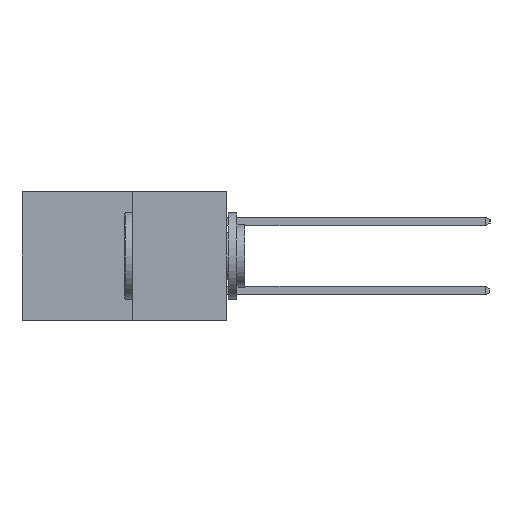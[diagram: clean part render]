
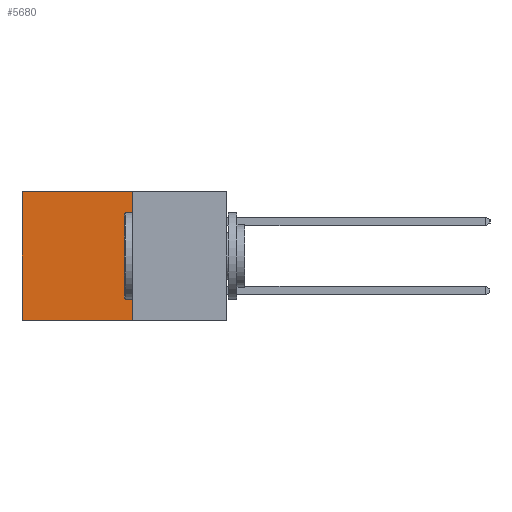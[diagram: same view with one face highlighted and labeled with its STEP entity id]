
A CAD part, left-side view. The second image highlights one B-rep face of the part: STEP entity #5680.
In plain terms, the highlighted planar face has unit normal (-1, 0, 0).
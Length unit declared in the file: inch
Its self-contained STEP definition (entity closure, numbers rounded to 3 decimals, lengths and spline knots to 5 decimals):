
#128 = DIRECTION ( 'NONE',  ( 0., 0., -1. ) ) ;
#725 = EDGE_LOOP ( 'NONE', ( #756, #8304, #2112, #6330 ) ) ;
#756 = ORIENTED_EDGE ( 'NONE', *, *, #2723, .T. ) ;
#822 = CARTESIAN_POINT ( 'NONE',  ( 0.277, 0.27, 0. ) ) ;
#1038 = FACE_OUTER_BOUND ( 'NONE', #725, .T. ) ;
#1588 = PLANE ( 'NONE',  #3209 ) ;
#1801 = VERTEX_POINT ( 'NONE', #3300 ) ;
#1844 = LINE ( 'NONE', #6355, #12254 ) ;
#2112 = ORIENTED_EDGE ( 'NONE', *, *, #11086, .F. ) ;
#2601 = DIRECTION ( 'NONE',  ( 0., 0., -1. ) ) ;
#2723 = EDGE_CURVE ( 'NONE', #10650, #10129, #11982, .T. ) ;
#3209 = AXIS2_PLACEMENT_3D ( 'NONE', #4567, #8621, #2601 ) ;
#3300 = CARTESIAN_POINT ( 'NONE',  ( 0.277, 0.27, 0. ) ) ;
#3557 = CARTESIAN_POINT ( 'NONE',  ( 0.277, 0.59, 0. ) ) ;
#4363 = VECTOR ( 'NONE', #128, 39.37008 ) ;
#4567 = CARTESIAN_POINT ( 'NONE',  ( 0.277, 0.27, -0.37 ) ) ;
#4668 = LINE ( 'NONE', #12145, #4363 ) ;
#5408 = LINE ( 'NONE', #822, #11142 ) ;
#5680 = ADVANCED_FACE ( 'NONE', ( #1038 ), #1588, .F. ) ;
#6177 = EDGE_CURVE ( 'NONE', #12588, #10129, #1844, .T. ) ;
#6278 = DIRECTION ( 'NONE',  ( 0., 0., -1. ) ) ;
#6330 = ORIENTED_EDGE ( 'NONE', *, *, #7717, .T. ) ;
#6355 = CARTESIAN_POINT ( 'NONE',  ( 0.277, 0.27, -0.37 ) ) ;
#6951 = CARTESIAN_POINT ( 'NONE',  ( 0.277, 0.59, -0.37 ) ) ;
#7717 = EDGE_CURVE ( 'NONE', #1801, #10650, #5408, .T. ) ;
#7829 = DIRECTION ( 'NONE',  ( 0., 1., 0. ) ) ;
#8223 = CARTESIAN_POINT ( 'NONE',  ( 0.277, 0.27, -0.37 ) ) ;
#8304 = ORIENTED_EDGE ( 'NONE', *, *, #6177, .F. ) ;
#8621 = DIRECTION ( 'NONE',  ( 1., 0., 0. ) ) ;
#9283 = VECTOR ( 'NONE', #6278, 39.37008 ) ;
#9831 = CARTESIAN_POINT ( 'NONE',  ( 0.277, 0.59, -0.37 ) ) ;
#10129 = VERTEX_POINT ( 'NONE', #9831 ) ;
#10650 = VERTEX_POINT ( 'NONE', #3557 ) ;
#11086 = EDGE_CURVE ( 'NONE', #1801, #12588, #4668, .T. ) ;
#11142 = VECTOR ( 'NONE', #7829, 39.37008 ) ;
#11982 = LINE ( 'NONE', #6951, #9283 ) ;
#12145 = CARTESIAN_POINT ( 'NONE',  ( 0.277, 0.27, -0.37 ) ) ;
#12254 = VECTOR ( 'NONE', #12432, 39.37008 ) ;
#12432 = DIRECTION ( 'NONE',  ( 0., 1., 0. ) ) ;
#12588 = VERTEX_POINT ( 'NONE', #8223 ) ;
